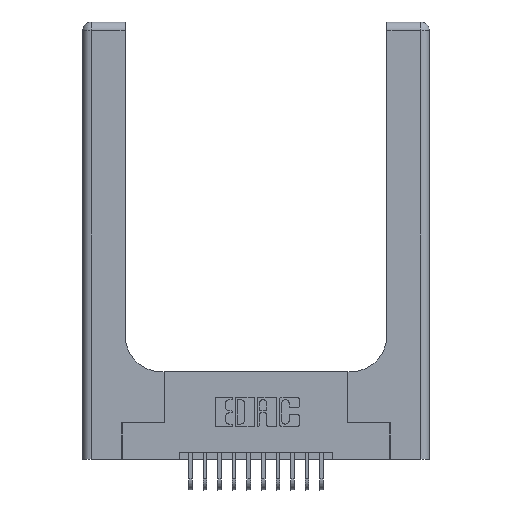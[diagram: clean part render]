
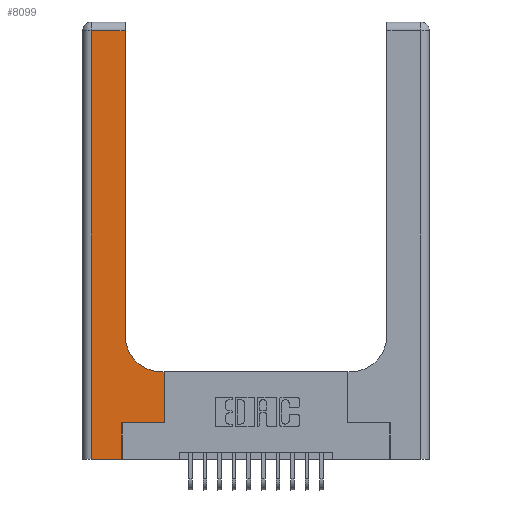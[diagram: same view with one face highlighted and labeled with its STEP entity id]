
A CAD part, top view. The second image highlights one B-rep face of the part: STEP entity #8099.
In plain terms, the highlighted planar face has unit normal (0, 0, 1).
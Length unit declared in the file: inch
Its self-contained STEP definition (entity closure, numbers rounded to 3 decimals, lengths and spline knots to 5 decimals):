
#441 = EDGE_CURVE ( 'NONE', #10320, #16829, #3593, .T. ) ;
#649 = ORIENTED_EDGE ( 'NONE', *, *, #7468, .T. ) ;
#733 = DIRECTION ( 'NONE',  ( 0., 1., 0. ) ) ;
#866 = CARTESIAN_POINT ( 'NONE',  ( 0.5585, 0.25, 0.37 ) ) ;
#909 = LINE ( 'NONE', #8143, #4457 ) ;
#1302 = EDGE_CURVE ( 'NONE', #12620, #6646, #15778, .T. ) ;
#1330 = VECTOR ( 'NONE', #8537, 39.37008 ) ;
#1862 = VERTEX_POINT ( 'NONE', #18854 ) ;
#2090 = DIRECTION ( 'NONE',  ( 0., 0., -1. ) ) ;
#2797 = DIRECTION ( 'NONE',  ( -1., 0., 0. ) ) ;
#2822 = LINE ( 'NONE', #4904, #16081 ) ;
#2987 = ORIENTED_EDGE ( 'NONE', *, *, #11101, .T. ) ;
#3593 = LINE ( 'NONE', #866, #10916 ) ;
#3888 = ORIENTED_EDGE ( 'NONE', *, *, #441, .T. ) ;
#4065 = VERTEX_POINT ( 'NONE', #18640 ) ;
#4131 = CARTESIAN_POINT ( 'NONE',  ( 0.2915, 0.85, 0.37 ) ) ;
#4278 = EDGE_CURVE ( 'NONE', #4811, #1862, #5433, .T. ) ;
#4457 = VECTOR ( 'NONE', #12390, 39.37008 ) ;
#4811 = VERTEX_POINT ( 'NONE', #4131 ) ;
#4904 = CARTESIAN_POINT ( 'NONE',  ( 0.06, 3., 0.37 ) ) ;
#5284 = CARTESIAN_POINT ( 'NONE',  ( 0.06, 2.94, 0.37 ) ) ;
#5299 = VERTEX_POINT ( 'NONE', #5284 ) ;
#5433 = LINE ( 'NONE', #17700, #16580 ) ;
#5810 = CARTESIAN_POINT ( 'NONE',  ( 0.5415, 0.6, 0.37 ) ) ;
#5857 = VECTOR ( 'NONE', #7842, 39.37008 ) ;
#6164 = EDGE_CURVE ( 'NONE', #16829, #9618, #10421, .T. ) ;
#6564 = VECTOR ( 'NONE', #10001, 39.37008 ) ;
#6646 = VERTEX_POINT ( 'NONE', #8535 ) ;
#7468 = EDGE_CURVE ( 'NONE', #6646, #4065, #16938, .T. ) ;
#7478 = CARTESIAN_POINT ( 'NONE',  ( 0.5585, 0.6, 0.37 ) ) ;
#7588 = DIRECTION ( 'NONE',  ( 0., 1., 0. ) ) ;
#7842 = DIRECTION ( 'NONE',  ( -1., 0., 0. ) ) ;
#7873 = EDGE_CURVE ( 'NONE', #9618, #4811, #18272, .T. ) ;
#8099 = ADVANCED_FACE ( 'NONE', ( #15130 ), #14478, .F. ) ;
#8143 = CARTESIAN_POINT ( 'NONE',  ( 0.269, 0.25, 0.37 ) ) ;
#8535 = CARTESIAN_POINT ( 'NONE',  ( 0.269, 0., 0.37 ) ) ;
#8537 = DIRECTION ( 'NONE',  ( 0., 1., 0. ) ) ;
#8548 = CARTESIAN_POINT ( 'NONE',  ( 0.2915, 0.6, 0.37 ) ) ;
#8790 = EDGE_LOOP ( 'NONE', ( #9065, #2987, #14674, #17740, #649, #12472, #3888, #18609, #9811 ) ) ;
#9065 = ORIENTED_EDGE ( 'NONE', *, *, #4278, .T. ) ;
#9297 = CARTESIAN_POINT ( 'NONE',  ( 0., 2.94, 0.37 ) ) ;
#9618 = VERTEX_POINT ( 'NONE', #5810 ) ;
#9811 = ORIENTED_EDGE ( 'NONE', *, *, #7873, .T. ) ;
#10001 = DIRECTION ( 'NONE',  ( -1., 0., 0. ) ) ;
#10151 = CARTESIAN_POINT ( 'NONE',  ( 0., 3., 0.37 ) ) ;
#10320 = VERTEX_POINT ( 'NONE', #18895 ) ;
#10421 = LINE ( 'NONE', #8548, #6564 ) ;
#10911 = CARTESIAN_POINT ( 'NONE',  ( 0.5415, 0.85, 0.37 ) ) ;
#10916 = VECTOR ( 'NONE', #733, 39.37008 ) ;
#11101 = EDGE_CURVE ( 'NONE', #1862, #5299, #17440, .T. ) ;
#11190 = EDGE_CURVE ( 'NONE', #4065, #10320, #909, .T. ) ;
#11584 = DIRECTION ( 'NONE',  ( 0., 0., -1. ) ) ;
#12386 = DIRECTION ( 'NONE',  ( 1., 0., 0. ) ) ;
#12390 = DIRECTION ( 'NONE',  ( 1., 0., 0. ) ) ;
#12394 = VECTOR ( 'NONE', #12954, 39.37008 ) ;
#12472 = ORIENTED_EDGE ( 'NONE', *, *, #11190, .T. ) ;
#12620 = VERTEX_POINT ( 'NONE', #15391 ) ;
#12954 = DIRECTION ( 'NONE',  ( 1., 0., 0. ) ) ;
#13401 = CARTESIAN_POINT ( 'NONE',  ( 0., 0., 0.37 ) ) ;
#13960 = AXIS2_PLACEMENT_3D ( 'NONE', #10151, #11584, #2797 ) ;
#14376 = CARTESIAN_POINT ( 'NONE',  ( 0.269, 0., 0.37 ) ) ;
#14478 = PLANE ( 'NONE',  #13960 ) ;
#14674 = ORIENTED_EDGE ( 'NONE', *, *, #16462, .T. ) ;
#15130 = FACE_OUTER_BOUND ( 'NONE', #8790, .T. ) ;
#15391 = CARTESIAN_POINT ( 'NONE',  ( 0.06, 0., 0.37 ) ) ;
#15778 = LINE ( 'NONE', #13401, #12394 ) ;
#16081 = VECTOR ( 'NONE', #16547, 39.37008 ) ;
#16462 = EDGE_CURVE ( 'NONE', #5299, #12620, #2822, .T. ) ;
#16547 = DIRECTION ( 'NONE',  ( 0., -1., 0. ) ) ;
#16580 = VECTOR ( 'NONE', #7588, 39.37008 ) ;
#16829 = VERTEX_POINT ( 'NONE', #7478 ) ;
#16938 = LINE ( 'NONE', #14376, #1330 ) ;
#17182 = AXIS2_PLACEMENT_3D ( 'NONE', #10911, #2090, #12386 ) ;
#17440 = LINE ( 'NONE', #9297, #5857 ) ;
#17700 = CARTESIAN_POINT ( 'NONE',  ( 0.2915, 3., 0.37 ) ) ;
#17740 = ORIENTED_EDGE ( 'NONE', *, *, #1302, .T. ) ;
#18272 = CIRCLE ( 'NONE', #17182, 0.25 ) ;
#18609 = ORIENTED_EDGE ( 'NONE', *, *, #6164, .T. ) ;
#18640 = CARTESIAN_POINT ( 'NONE',  ( 0.269, 0.25, 0.37 ) ) ;
#18854 = CARTESIAN_POINT ( 'NONE',  ( 0.2915, 2.94, 0.37 ) ) ;
#18895 = CARTESIAN_POINT ( 'NONE',  ( 0.5585, 0.25, 0.37 ) ) ;
